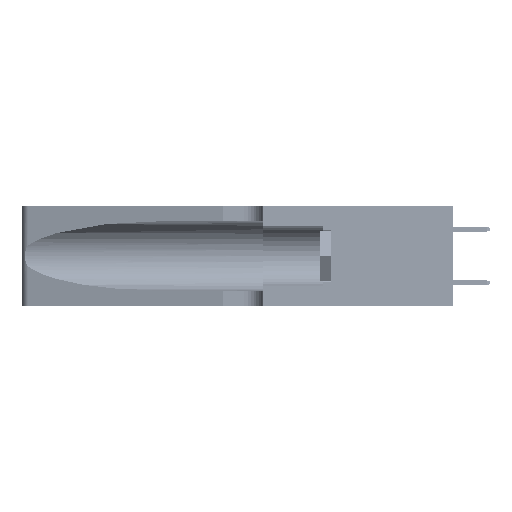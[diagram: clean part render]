
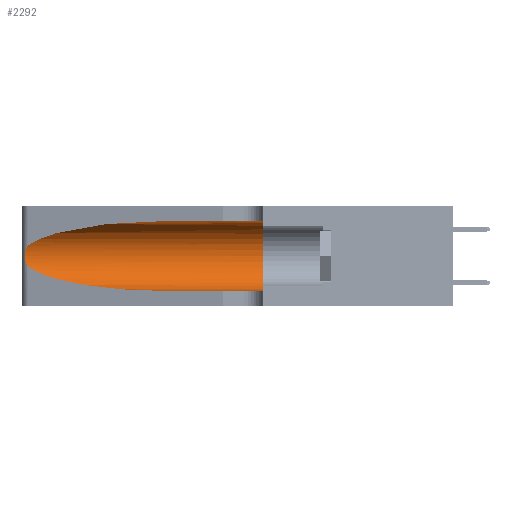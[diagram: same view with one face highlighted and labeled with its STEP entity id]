
A CAD part, left-side view. The second image highlights one B-rep face of the part: STEP entity #2292.
In plain terms, the highlighted cylindrical face has radius 3.308 mm (diameter 6.617 mm), a partial arc.
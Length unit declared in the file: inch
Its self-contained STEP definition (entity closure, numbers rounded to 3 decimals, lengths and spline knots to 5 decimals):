
#772 = VERTEX_POINT ( 'NONE', #7663 ) ;
#1886 = CIRCLE ( 'NONE', #42751, 0.13025 ) ;
#2199 = DIRECTION ( 'NONE',  ( 0., 1., 0. ) ) ;
#2292 = ADVANCED_FACE ( 'NONE', ( #30800 ), #31149, .F. ) ;
#2930 = CARTESIAN_POINT ( 'NONE',  ( 0.25487, 1.22718, 0.14631 ) ) ;
#3894 = CARTESIAN_POINT ( 'NONE',  ( 0.26017, 1.23833, 0.17102 ) ) ;
#4255 = CARTESIAN_POINT ( 'NONE',  ( 0.2373, 1.15595, 0.28018 ) ) ;
#4400 = VECTOR ( 'NONE', #39332, 39.37008 ) ;
#6106 = CARTESIAN_POINT ( 'NONE',  ( 0.25789, 1.23486, 0.15765 ) ) ;
#6526 = ORIENTED_EDGE ( 'NONE', *, *, #32594, .T. ) ;
#6637 = CARTESIAN_POINT ( 'NONE',  ( 0.25856, 1.23593, 0.16098 ) ) ;
#7663 = CARTESIAN_POINT ( 'NONE',  ( 0.25487, 1.22718, 0.22369 ) ) ;
#8574 = CARTESIAN_POINT ( 'NONE',  ( 0.1305, 1.61858, 0.05475 ) ) ;
#11949 = DIRECTION ( 'NONE',  ( 0., -1., 0. ) ) ;
#12110 = ORIENTED_EDGE ( 'NONE', *, *, #30667, .T. ) ;
#13535 = CARTESIAN_POINT ( 'NONE',  ( 0.18966, 0.96281, 0.05475 ) ) ;
#13969 = VERTEX_POINT ( 'NONE', #37341 ) ;
#14064 = CARTESIAN_POINT ( 'NONE',  ( 0.1305, 0.72297, 0.05475 ) ) ;
#14202 = CARTESIAN_POINT ( 'NONE',  ( 0.25555, 1.22993, 0.14849 ) ) ;
#14446 = CARTESIAN_POINT ( 'NONE',  ( 0.25854, 1.2359, 0.20912 ) ) ;
#15481 = DIRECTION ( 'NONE',  ( 0., -1., 0. ) ) ;
#18132 = DIRECTION ( 'NONE',  ( 0., 0., 1. ) ) ;
#18346 = CARTESIAN_POINT ( 'NONE',  ( 0.25787, 1.23484, 0.2124 ) ) ;
#19489 = LINE ( 'NONE', #23673, #4400 ) ;
#20423 = CARTESIAN_POINT ( 'NONE',  ( 0.18966, 0.96281, 0.31525 ) ) ;
#22323 = CARTESIAN_POINT ( 'NONE',  ( 0.1305, 0.35, 0.185 ) ) ;
#22343 = VERTEX_POINT ( 'NONE', #37394 ) ;
#22895 = ORIENTED_EDGE ( 'NONE', *, *, #36322, .T. ) ;
#23066 = CARTESIAN_POINT ( 'NONE',  ( 0.1305, 1.61858, 0.185 ) ) ;
#23310 = EDGE_LOOP ( 'NONE', ( #12110, #22895, #35595, #6526, #41648, #23494 ) ) ;
#23494 = ORIENTED_EDGE ( 'NONE', *, *, #28236, .F. ) ;
#23673 = CARTESIAN_POINT ( 'NONE',  ( 0.1305, 1.61858, 0.31525 ) ) ;
#26453 = CARTESIAN_POINT ( 'NONE',  ( 0.26018, 1.23835, 0.19895 ) ) ;
#27547 = CARTESIAN_POINT ( 'NONE',  ( 0.1305, 0.72297, 0.05475 ) ) ;
#28116 = LINE ( 'NONE', #8574, #35368 ) ;
#28236 = EDGE_CURVE ( 'NONE', #13969, #36810, #19489, .T. ) ;
#30667 = EDGE_CURVE ( 'NONE', #13969, #772, #46651, .T. ) ;
#30800 = FACE_OUTER_BOUND ( 'NONE', #23310, .T. ) ;
#31149 = CYLINDRICAL_SURFACE ( 'NONE', #39074, 0.13025 ) ;
#32594 = EDGE_CURVE ( 'NONE', #47624, #48537, #28116, .T. ) ;
#34002 = CARTESIAN_POINT ( 'NONE',  ( 0.25487, 1.22718, 0.22369 ) ) ;
#34265 = CARTESIAN_POINT ( 'NONE',  ( 0.25639, 1.23186, 0.15144 ) ) ;
#35230 = CARTESIAN_POINT ( 'NONE',  ( 0.1305, 0.35, 0.05475 ) ) ;
#35368 = VECTOR ( 'NONE', #11949, 39.37008 ) ;
#35554 = DIRECTION ( 'NONE',  ( 0., 0., -1. ) ) ;
#35595 = ORIENTED_EDGE ( 'NONE', *, *, #50199, .T. ) ;
#36322 = EDGE_CURVE ( 'NONE', #772, #22343, #47254, .T. ) ;
#36810 = VERTEX_POINT ( 'NONE', #38377 ) ;
#37341 = CARTESIAN_POINT ( 'NONE',  ( 0.1305, 0.72297, 0.31525 ) ) ;
#37394 = CARTESIAN_POINT ( 'NONE',  ( 0.25487, 1.22718, 0.14631 ) ) ;
#38377 = CARTESIAN_POINT ( 'NONE',  ( 0.1305, 0.35, 0.31525 ) ) ;
#38453 = CARTESIAN_POINT ( 'NONE',  ( 0.25555, 1.22994, 0.2215 ) ) ;
#38706 = CARTESIAN_POINT ( 'NONE',  ( 0.26075, 1.23896, 0.19203 ) ) ;
#39074 = AXIS2_PLACEMENT_3D ( 'NONE', #23066, #15481, #35554 ) ;
#39332 = DIRECTION ( 'NONE',  ( 0., -1., 0. ) ) ;
#39642 = CARTESIAN_POINT ( 'NONE',  ( 0.26075, 1.23896, 0.178 ) ) ;
#41252 = EDGE_CURVE ( 'NONE', #36810, #48537, #1886, .T. ) ;
#41648 = ORIENTED_EDGE ( 'NONE', *, *, #41252, .F. ) ;
#42751 = AXIS2_PLACEMENT_3D ( 'NONE', #22323, #2199, #18132 ) ;
#43932 = CARTESIAN_POINT ( 'NONE',  ( 0.1305, 0.72297, 0.31525 ) ) ;
#45284 =( BOUNDED_CURVE ( )  B_SPLINE_CURVE ( 3, ( #45369, #45885, #13535, #14064 ),
 .UNSPECIFIED., .F., .T. ) 
 B_SPLINE_CURVE_WITH_KNOTS ( ( 4, 4 ),
 ( 3.44316, 4.71239 ),
 .UNSPECIFIED. ) 
 CURVE ( )  GEOMETRIC_REPRESENTATION_ITEM ( )  RATIONAL_B_SPLINE_CURVE ( ( 1., 0.87, 0.87, 1. ) ) 
 REPRESENTATION_ITEM ( '' )  );
#45369 = CARTESIAN_POINT ( 'NONE',  ( 0.25487, 1.22718, 0.14631 ) ) ;
#45885 = CARTESIAN_POINT ( 'NONE',  ( 0.2373, 1.15595, 0.08982 ) ) ;
#46651 =( BOUNDED_CURVE ( )  B_SPLINE_CURVE ( 3, ( #43932, #20423, #4255, #48096 ),
 .UNSPECIFIED., .F., .T. ) 
 B_SPLINE_CURVE_WITH_KNOTS ( ( 4, 4 ),
 ( 1.5708, 2.84003 ),
 .UNSPECIFIED. ) 
 CURVE ( )  GEOMETRIC_REPRESENTATION_ITEM ( )  RATIONAL_B_SPLINE_CURVE ( ( 1., 0.87, 0.87, 1. ) ) 
 REPRESENTATION_ITEM ( '' )  );
#47254 = B_SPLINE_CURVE_WITH_KNOTS ( 'NONE', 3,
 ( #34002, #38453, #49952, #18346, #14446, #26453, #38706, #39642, #3894, #6637, #6106, #34265, #14202, #2930 ),
 .UNSPECIFIED., .F., .F.,
 ( 4, 2, 2, 2, 2, 2, 4 ),
 ( 0., 0.00027, 0.00053, 0.00107, 0.0016, 0.00187, 0.00214 ),
 .UNSPECIFIED. ) ;
#47624 = VERTEX_POINT ( 'NONE', #27547 ) ;
#48096 = CARTESIAN_POINT ( 'NONE',  ( 0.25487, 1.22718, 0.22369 ) ) ;
#48537 = VERTEX_POINT ( 'NONE', #35230 ) ;
#49952 = CARTESIAN_POINT ( 'NONE',  ( 0.25639, 1.23184, 0.21858 ) ) ;
#50199 = EDGE_CURVE ( 'NONE', #22343, #47624, #45284, .T. ) ;
